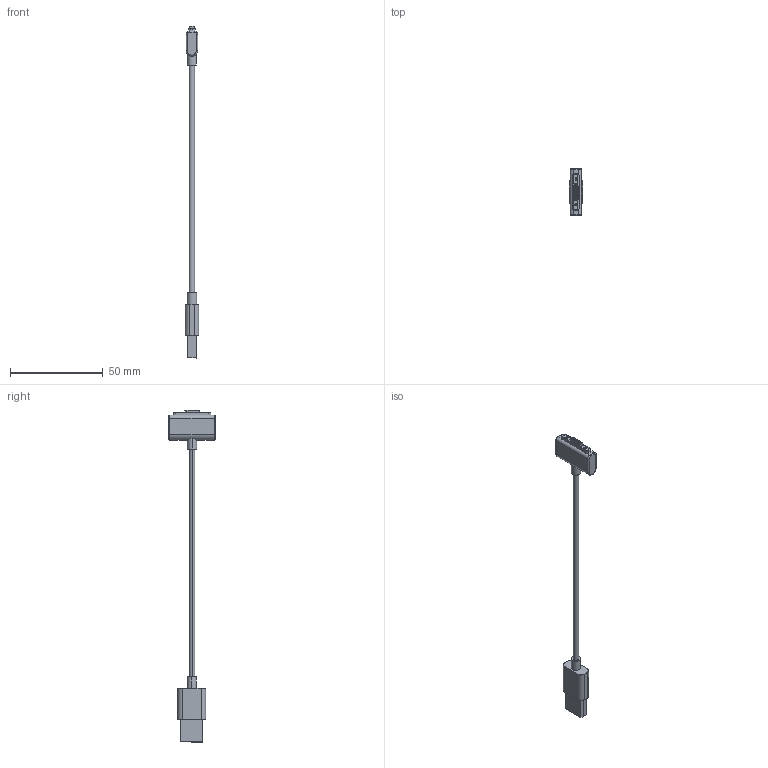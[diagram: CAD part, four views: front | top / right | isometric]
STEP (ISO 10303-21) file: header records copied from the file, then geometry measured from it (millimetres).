
FILE_DESCRIPTION (( 'STEP AP214' ), '1' );
FILE_NAME ('687K0412A501100.STEP', '2023-05-01T18:56:37', ( '' ), ( '' ), 'SwSTEP 2.0', 'SolidWorks 2020', '' );
FILE_SCHEMA (( 'AUTOMOTIVE_DESIGN' ));
Length unit declared in the file: millimetre
Products named in the file (1): 687K0412A501100
Bounding box: 7.2 x 25.3 x 179.17 mm (x, y, z)
Volume: 5281.1 mm3; surface area: 4403.1 mm2
Topology: 6 solids, 6 shells, 275 faces, 652 edges, 408 vertices
Faces by surface type: plane 151, cylinder 74, cone 19, torus 17, bspline 14
Entity records: 11598 total; most frequent: CARTESIAN_POINT 2230, DIRECTION 1319, ORIENTED_EDGE 1288, EDGE_CURVE 644, AXIS2_PLACEMENT_3D 447, VECTOR 425, LINE 425, VERTEX_POINT 408
